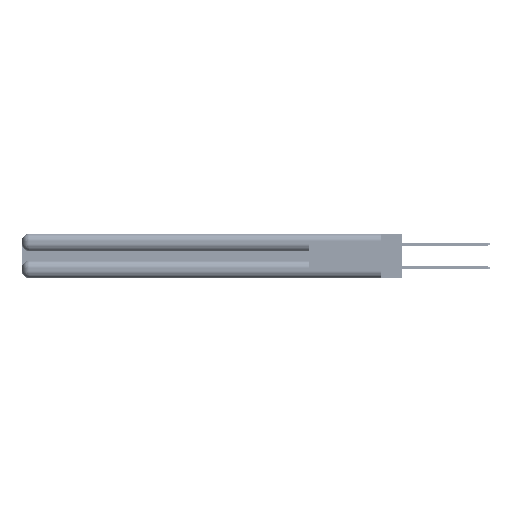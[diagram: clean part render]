
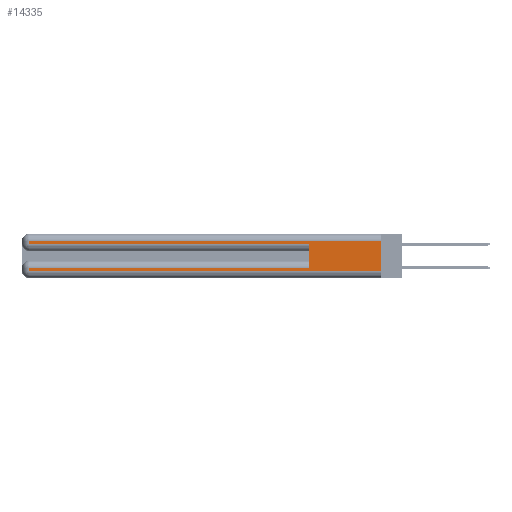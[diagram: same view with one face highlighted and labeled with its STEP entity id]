
A CAD part, left-side view. The second image highlights one B-rep face of the part: STEP entity #14335.
In plain terms, the highlighted planar face has unit normal (-1, 0, 0).
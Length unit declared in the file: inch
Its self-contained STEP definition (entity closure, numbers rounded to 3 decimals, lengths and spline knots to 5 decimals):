
#40 = VERTEX_POINT ( 'NONE', #45833 ) ;
#1287 = EDGE_CURVE ( 'NONE', #22567, #32050, #41510, .T. ) ;
#1479 = LINE ( 'NONE', #8601, #23677 ) ;
#2024 = DIRECTION ( 'NONE',  ( 0., 1., 0. ) ) ;
#3097 = LINE ( 'NONE', #19115, #44740 ) ;
#3363 = VERTEX_POINT ( 'NONE', #12483 ) ;
#3739 = ORIENTED_EDGE ( 'NONE', *, *, #20728, .T. ) ;
#5647 = CARTESIAN_POINT ( 'NONE',  ( 0., 0., 0.37 ) ) ;
#7581 = ORIENTED_EDGE ( 'NONE', *, *, #28105, .F. ) ;
#7694 = CARTESIAN_POINT ( 'NONE',  ( 0., 0., 0.37 ) ) ;
#7895 = PLANE ( 'NONE',  #48046 ) ;
#8409 = DIRECTION ( 'NONE',  ( 0., 0., -1. ) ) ;
#8601 = CARTESIAN_POINT ( 'NONE',  ( 0., 2.94, 0.37 ) ) ;
#8807 = LINE ( 'NONE', #30814, #21582 ) ;
#9954 = LINE ( 'NONE', #40512, #15303 ) ;
#10329 = EDGE_CURVE ( 'NONE', #51960, #40, #39103, .T. ) ;
#10434 = CARTESIAN_POINT ( 'NONE',  ( 0., 0., 0.085 ) ) ;
#12020 = EDGE_CURVE ( 'NONE', #53743, #32291, #1479, .T. ) ;
#12081 = CARTESIAN_POINT ( 'NONE',  ( 0., 2.94, 0.31 ) ) ;
#12483 = CARTESIAN_POINT ( 'NONE',  ( 0., 2.94, 0.06 ) ) ;
#14095 = DIRECTION ( 'NONE',  ( 0., 0., -1. ) ) ;
#14335 = ADVANCED_FACE ( 'NONE', ( #23360 ), #7895, .F. ) ;
#15303 = VECTOR ( 'NONE', #2024, 39.37008 ) ;
#15515 = DIRECTION ( 'NONE',  ( 0., 1., 0. ) ) ;
#18328 = LINE ( 'NONE', #45756, #25036 ) ;
#18520 = EDGE_CURVE ( 'NONE', #3363, #40, #40582, .T. ) ;
#18707 = VECTOR ( 'NONE', #15515, 39.37008 ) ;
#19115 = CARTESIAN_POINT ( 'NONE',  ( 0., 0.6, 0.145 ) ) ;
#19680 = DIRECTION ( 'NONE',  ( 0., -1., 0. ) ) ;
#20307 = DIRECTION ( 'NONE',  ( 0., 0., -1. ) ) ;
#20728 = EDGE_CURVE ( 'NONE', #32050, #3363, #8807, .T. ) ;
#21054 = ORIENTED_EDGE ( 'NONE', *, *, #18520, .T. ) ;
#21237 = ORIENTED_EDGE ( 'NONE', *, *, #39885, .T. ) ;
#21582 = VECTOR ( 'NONE', #25566, 39.37008 ) ;
#22226 = CARTESIAN_POINT ( 'NONE',  ( 0., 0.6, 0.285 ) ) ;
#22567 = VERTEX_POINT ( 'NONE', #46058 ) ;
#23345 = VERTEX_POINT ( 'NONE', #22226 ) ;
#23360 = FACE_OUTER_BOUND ( 'NONE', #24693, .T. ) ;
#23677 = VECTOR ( 'NONE', #8409, 39.37008 ) ;
#24143 = CARTESIAN_POINT ( 'NONE',  ( 0., 0., 0.06 ) ) ;
#24693 = EDGE_LOOP ( 'NONE', ( #30055, #21237, #51373, #45711, #7581, #42132, #3739, #21054 ) ) ;
#25036 = VECTOR ( 'NONE', #49887, 39.37008 ) ;
#25566 = DIRECTION ( 'NONE',  ( 0., 0., -1. ) ) ;
#26021 = CARTESIAN_POINT ( 'NONE',  ( 0., 0., 0.31 ) ) ;
#28105 = EDGE_CURVE ( 'NONE', #22567, #23345, #3097, .T. ) ;
#30055 = ORIENTED_EDGE ( 'NONE', *, *, #10329, .F. ) ;
#30118 = CARTESIAN_POINT ( 'NONE',  ( 0., 2.94, 0.085 ) ) ;
#30814 = CARTESIAN_POINT ( 'NONE',  ( 0., 2.94, 0.37 ) ) ;
#32050 = VERTEX_POINT ( 'NONE', #30118 ) ;
#32291 = VERTEX_POINT ( 'NONE', #35165 ) ;
#33112 = EDGE_CURVE ( 'NONE', #32291, #23345, #18328, .T. ) ;
#34375 = VECTOR ( 'NONE', #14095, 39.37008 ) ;
#35165 = CARTESIAN_POINT ( 'NONE',  ( 0., 2.94, 0.285 ) ) ;
#35891 = VECTOR ( 'NONE', #19680, 39.37008 ) ;
#39103 = LINE ( 'NONE', #5647, #34375 ) ;
#39885 = EDGE_CURVE ( 'NONE', #51960, #53743, #9954, .T. ) ;
#40512 = CARTESIAN_POINT ( 'NONE',  ( 0., 0., 0.31 ) ) ;
#40582 = LINE ( 'NONE', #24143, #35891 ) ;
#41510 = LINE ( 'NONE', #10434, #18707 ) ;
#42132 = ORIENTED_EDGE ( 'NONE', *, *, #1287, .T. ) ;
#44740 = VECTOR ( 'NONE', #45175, 39.37008 ) ;
#45175 = DIRECTION ( 'NONE',  ( 0., 0., 1. ) ) ;
#45711 = ORIENTED_EDGE ( 'NONE', *, *, #33112, .T. ) ;
#45756 = CARTESIAN_POINT ( 'NONE',  ( 0., 0., 0.285 ) ) ;
#45833 = CARTESIAN_POINT ( 'NONE',  ( 0., 0., 0.06 ) ) ;
#46058 = CARTESIAN_POINT ( 'NONE',  ( 0., 0.6, 0.085 ) ) ;
#48046 = AXIS2_PLACEMENT_3D ( 'NONE', #7694, #50516, #20307 ) ;
#49887 = DIRECTION ( 'NONE',  ( 0., -1., 0. ) ) ;
#50516 = DIRECTION ( 'NONE',  ( 1., 0., 0. ) ) ;
#51373 = ORIENTED_EDGE ( 'NONE', *, *, #12020, .T. ) ;
#51960 = VERTEX_POINT ( 'NONE', #26021 ) ;
#53743 = VERTEX_POINT ( 'NONE', #12081 ) ;
